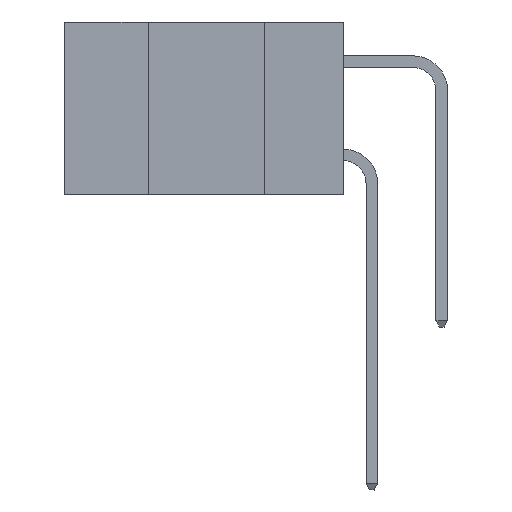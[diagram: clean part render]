
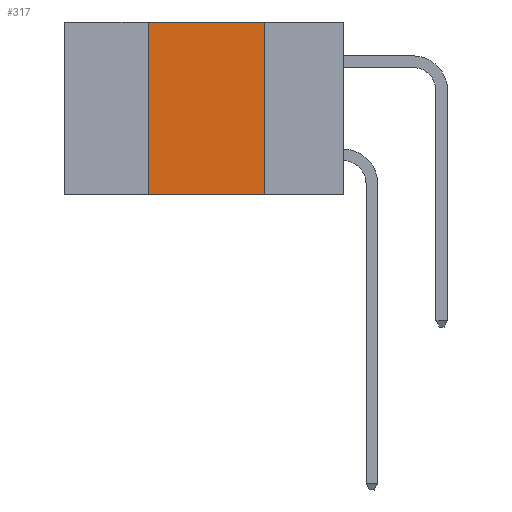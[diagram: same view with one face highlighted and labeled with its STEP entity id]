
A CAD part, left-side view. The second image highlights one B-rep face of the part: STEP entity #317.
In plain terms, the highlighted planar face has unit normal (-1, 0, 0).
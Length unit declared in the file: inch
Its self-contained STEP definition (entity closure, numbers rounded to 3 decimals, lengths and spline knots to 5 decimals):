
#38 = CARTESIAN_POINT ( 'NONE',  ( 0., 0.6, -0.37 ) ) ;
#317 = ADVANCED_FACE ( 'NONE', ( #5872 ), #4789, .F. ) ;
#598 = ORIENTED_EDGE ( 'NONE', *, *, #11600, .F. ) ;
#686 = EDGE_CURVE ( 'NONE', #13026, #13111, #19708, .T. ) ;
#712 = DIRECTION ( 'NONE',  ( 0., 0., -1. ) ) ;
#796 = DIRECTION ( 'NONE',  ( 1., 0., 0. ) ) ;
#1340 = LINE ( 'NONE', #38, #20700 ) ;
#1508 = CARTESIAN_POINT ( 'NONE',  ( 0., 0.17, 0. ) ) ;
#2079 = LINE ( 'NONE', #1508, #5372 ) ;
#3173 = DIRECTION ( 'NONE',  ( 0., 0., -1. ) ) ;
#3819 = EDGE_LOOP ( 'NONE', ( #598, #10192, #5886, #4273 ) ) ;
#4273 = ORIENTED_EDGE ( 'NONE', *, *, #11011, .T. ) ;
#4387 = CARTESIAN_POINT ( 'NONE',  ( 0., 0.17, -0.37 ) ) ;
#4789 = PLANE ( 'NONE',  #19309 ) ;
#4823 = LINE ( 'NONE', #15137, #13903 ) ;
#5372 = VECTOR ( 'NONE', #3173, 39.37008 ) ;
#5872 = FACE_OUTER_BOUND ( 'NONE', #3819, .T. ) ;
#5886 = ORIENTED_EDGE ( 'NONE', *, *, #15152, .F. ) ;
#6851 = VECTOR ( 'NONE', #12620, 39.37008 ) ;
#10192 = ORIENTED_EDGE ( 'NONE', *, *, #686, .F. ) ;
#11011 = EDGE_CURVE ( 'NONE', #11168, #15376, #1340, .T. ) ;
#11168 = VERTEX_POINT ( 'NONE', #19785 ) ;
#11486 = CARTESIAN_POINT ( 'NONE',  ( 0., 0.17, 0. ) ) ;
#11600 = EDGE_CURVE ( 'NONE', #13111, #15376, #2079, .T. ) ;
#12239 = CARTESIAN_POINT ( 'NONE',  ( 0., 0.6, 0. ) ) ;
#12620 = DIRECTION ( 'NONE',  ( 0., -1., 0. ) ) ;
#13026 = VERTEX_POINT ( 'NONE', #14563 ) ;
#13111 = VERTEX_POINT ( 'NONE', #11486 ) ;
#13903 = VECTOR ( 'NONE', #16743, 39.37008 ) ;
#14563 = CARTESIAN_POINT ( 'NONE',  ( 0., 0.42, 0. ) ) ;
#14612 = DIRECTION ( 'NONE',  ( 0., -1., 0. ) ) ;
#15137 = CARTESIAN_POINT ( 'NONE',  ( 0., 0.42, 0. ) ) ;
#15152 = EDGE_CURVE ( 'NONE', #11168, #13026, #4823, .T. ) ;
#15376 = VERTEX_POINT ( 'NONE', #4387 ) ;
#16743 = DIRECTION ( 'NONE',  ( 0., 0., 1. ) ) ;
#18393 = CARTESIAN_POINT ( 'NONE',  ( 0., 0.6, 0. ) ) ;
#19309 = AXIS2_PLACEMENT_3D ( 'NONE', #12239, #796, #712 ) ;
#19708 = LINE ( 'NONE', #18393, #6851 ) ;
#19785 = CARTESIAN_POINT ( 'NONE',  ( 0., 0.42, -0.37 ) ) ;
#20700 = VECTOR ( 'NONE', #14612, 39.37008 ) ;
